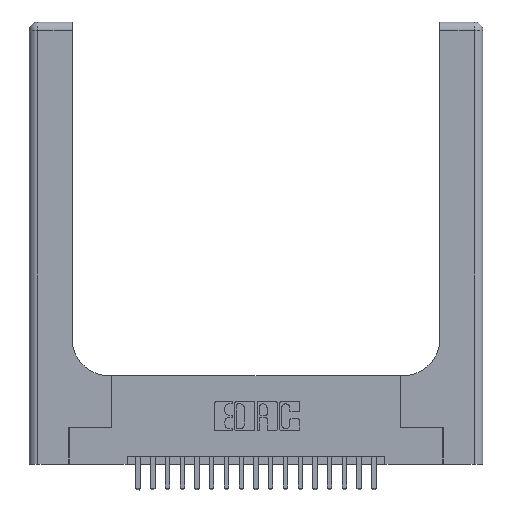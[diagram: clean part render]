
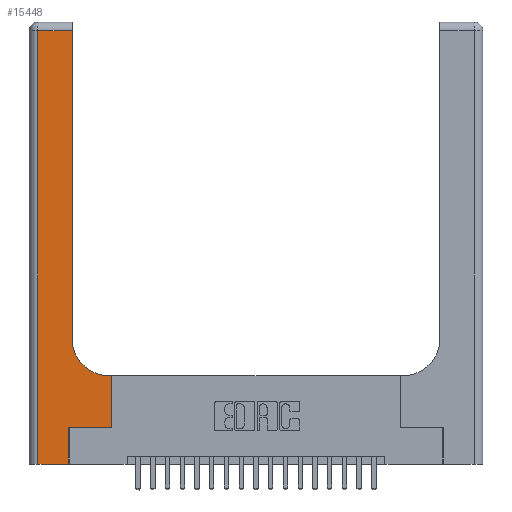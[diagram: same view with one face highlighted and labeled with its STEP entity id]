
A CAD part, top view. The second image highlights one B-rep face of the part: STEP entity #15448.
In plain terms, the highlighted planar face has unit normal (0, 0, 1).
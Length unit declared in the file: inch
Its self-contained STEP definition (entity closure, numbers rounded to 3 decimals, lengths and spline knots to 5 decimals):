
#11 = VERTEX_POINT ( 'NONE', #3350 ) ;
#536 = DIRECTION ( 'NONE',  ( 1., 0., 0. ) ) ;
#657 = VECTOR ( 'NONE', #1278, 39.37008 ) ;
#685 = CARTESIAN_POINT ( 'NONE',  ( 0.5585, 0.25, 0.37 ) ) ;
#945 = VERTEX_POINT ( 'NONE', #5257 ) ;
#1278 = DIRECTION ( 'NONE',  ( 0., 1., 0. ) ) ;
#1548 = CARTESIAN_POINT ( 'NONE',  ( 0.06, 2.94, 0.37 ) ) ;
#1730 = LINE ( 'NONE', #13790, #21459 ) ;
#1875 = LINE ( 'NONE', #18277, #7208 ) ;
#2216 = CARTESIAN_POINT ( 'NONE',  ( 0.269, 0., 0.37 ) ) ;
#2603 = PLANE ( 'NONE',  #17721 ) ;
#2684 = DIRECTION ( 'NONE',  ( 0., 0., -1. ) ) ;
#2720 = ORIENTED_EDGE ( 'NONE', *, *, #10868, .T. ) ;
#3082 = CARTESIAN_POINT ( 'NONE',  ( 0.2915, 0.6, 0.37 ) ) ;
#3350 = CARTESIAN_POINT ( 'NONE',  ( 0.5415, 0.6, 0.37 ) ) ;
#3404 = VERTEX_POINT ( 'NONE', #13036 ) ;
#3476 = EDGE_CURVE ( 'NONE', #11177, #6563, #1875, .T. ) ;
#3590 = DIRECTION ( 'NONE',  ( 1., 0., 0. ) ) ;
#3927 = VECTOR ( 'NONE', #7690, 39.37008 ) ;
#4179 = LINE ( 'NONE', #4472, #3927 ) ;
#4402 = CARTESIAN_POINT ( 'NONE',  ( 0., 3., 0.37 ) ) ;
#4472 = CARTESIAN_POINT ( 'NONE',  ( 0., 2.94, 0.37 ) ) ;
#4765 = ORIENTED_EDGE ( 'NONE', *, *, #12842, .T. ) ;
#4874 = LINE ( 'NONE', #8393, #9401 ) ;
#5257 = CARTESIAN_POINT ( 'NONE',  ( 0.2915, 0.85, 0.37 ) ) ;
#5485 = ORIENTED_EDGE ( 'NONE', *, *, #21598, .T. ) ;
#5945 = VERTEX_POINT ( 'NONE', #19988 ) ;
#5999 = CARTESIAN_POINT ( 'NONE',  ( 0.269, 0.25, 0.37 ) ) ;
#6498 = LINE ( 'NONE', #8190, #657 ) ;
#6563 = VERTEX_POINT ( 'NONE', #5999 ) ;
#7208 = VECTOR ( 'NONE', #10075, 39.37008 ) ;
#7327 = CIRCLE ( 'NONE', #7578, 0.25 ) ;
#7578 = AXIS2_PLACEMENT_3D ( 'NONE', #12353, #15716, #536 ) ;
#7667 = EDGE_CURVE ( 'NONE', #945, #3404, #6498, .T. ) ;
#7690 = DIRECTION ( 'NONE',  ( -1., 0., 0. ) ) ;
#8190 = CARTESIAN_POINT ( 'NONE',  ( 0.2915, 3., 0.37 ) ) ;
#8393 = CARTESIAN_POINT ( 'NONE',  ( 0.269, 0.25, 0.37 ) ) ;
#8714 = DIRECTION ( 'NONE',  ( 0., 1., 0. ) ) ;
#9401 = VECTOR ( 'NONE', #22011, 39.37008 ) ;
#9856 = ORIENTED_EDGE ( 'NONE', *, *, #19491, .T. ) ;
#10075 = DIRECTION ( 'NONE',  ( 0., 1., 0. ) ) ;
#10580 = CARTESIAN_POINT ( 'NONE',  ( 0.5585, 0.6, 0.37 ) ) ;
#10868 = EDGE_CURVE ( 'NONE', #3404, #16365, #4179, .T. ) ;
#11177 = VERTEX_POINT ( 'NONE', #2216 ) ;
#11789 = ORIENTED_EDGE ( 'NONE', *, *, #16741, .T. ) ;
#12353 = CARTESIAN_POINT ( 'NONE',  ( 0.5415, 0.85, 0.37 ) ) ;
#12842 = EDGE_CURVE ( 'NONE', #11, #945, #7327, .T. ) ;
#13036 = CARTESIAN_POINT ( 'NONE',  ( 0.2915, 2.94, 0.37 ) ) ;
#13244 = LINE ( 'NONE', #19347, #21248 ) ;
#13790 = CARTESIAN_POINT ( 'NONE',  ( 0.5585, 0.25, 0.37 ) ) ;
#14390 = VERTEX_POINT ( 'NONE', #10580 ) ;
#14714 = DIRECTION ( 'NONE',  ( -1., 0., 0. ) ) ;
#15448 = ADVANCED_FACE ( 'NONE', ( #19849 ), #2603, .F. ) ;
#15716 = DIRECTION ( 'NONE',  ( 0., 0., -1. ) ) ;
#15734 = ORIENTED_EDGE ( 'NONE', *, *, #16073, .T. ) ;
#16073 = EDGE_CURVE ( 'NONE', #5945, #11177, #19826, .T. ) ;
#16357 = CARTESIAN_POINT ( 'NONE',  ( 0., 0., 0.37 ) ) ;
#16365 = VERTEX_POINT ( 'NONE', #1548 ) ;
#16376 = EDGE_CURVE ( 'NONE', #6563, #17656, #4874, .T. ) ;
#16741 = EDGE_CURVE ( 'NONE', #14390, #11, #18446, .T. ) ;
#17566 = DIRECTION ( 'NONE',  ( 0., -1., 0. ) ) ;
#17656 = VERTEX_POINT ( 'NONE', #685 ) ;
#17676 = VECTOR ( 'NONE', #3590, 39.37008 ) ;
#17721 = AXIS2_PLACEMENT_3D ( 'NONE', #4402, #2684, #14714 ) ;
#18230 = DIRECTION ( 'NONE',  ( -1., 0., 0. ) ) ;
#18277 = CARTESIAN_POINT ( 'NONE',  ( 0.269, 0., 0.37 ) ) ;
#18446 = LINE ( 'NONE', #3082, #19502 ) ;
#18902 = ORIENTED_EDGE ( 'NONE', *, *, #3476, .T. ) ;
#19347 = CARTESIAN_POINT ( 'NONE',  ( 0.06, 3., 0.37 ) ) ;
#19491 = EDGE_CURVE ( 'NONE', #16365, #5945, #13244, .T. ) ;
#19502 = VECTOR ( 'NONE', #18230, 39.37008 ) ;
#19826 = LINE ( 'NONE', #16357, #17676 ) ;
#19849 = FACE_OUTER_BOUND ( 'NONE', #20512, .T. ) ;
#19988 = CARTESIAN_POINT ( 'NONE',  ( 0.06, 0., 0.37 ) ) ;
#20512 = EDGE_LOOP ( 'NONE', ( #21846, #2720, #9856, #15734, #18902, #20607, #5485, #11789, #4765 ) ) ;
#20607 = ORIENTED_EDGE ( 'NONE', *, *, #16376, .T. ) ;
#21248 = VECTOR ( 'NONE', #17566, 39.37008 ) ;
#21459 = VECTOR ( 'NONE', #8714, 39.37008 ) ;
#21598 = EDGE_CURVE ( 'NONE', #17656, #14390, #1730, .T. ) ;
#21846 = ORIENTED_EDGE ( 'NONE', *, *, #7667, .T. ) ;
#22011 = DIRECTION ( 'NONE',  ( 1., 0., 0. ) ) ;
